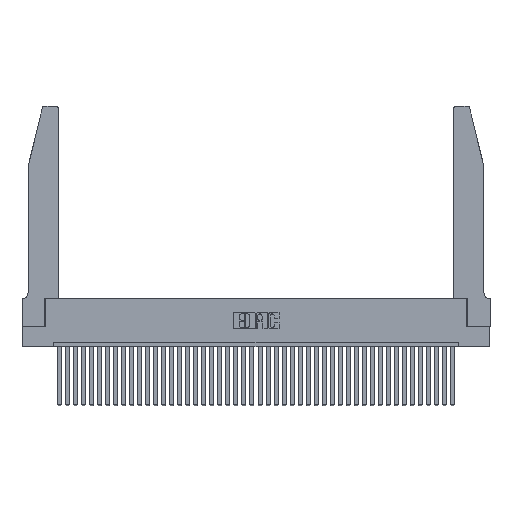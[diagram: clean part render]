
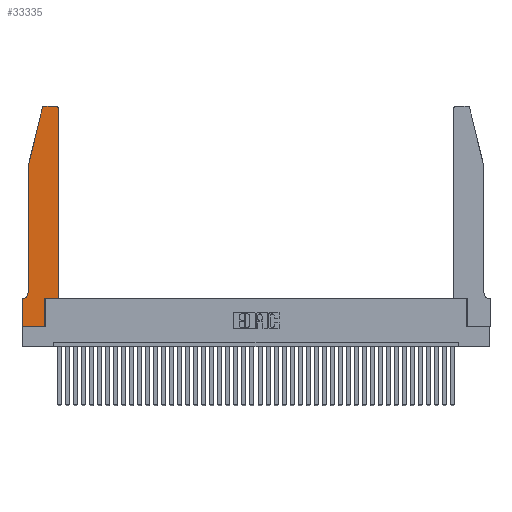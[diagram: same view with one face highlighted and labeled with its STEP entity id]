
A CAD part, top view. The second image highlights one B-rep face of the part: STEP entity #33335.
In plain terms, the highlighted planar face has unit normal (0, 0, 1).
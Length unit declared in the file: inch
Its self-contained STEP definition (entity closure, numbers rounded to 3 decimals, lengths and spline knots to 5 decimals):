
#812 = VERTEX_POINT ( 'NONE', #20611 ) ;
#815 = EDGE_CURVE ( 'NONE', #19528, #30898, #35516, .T. ) ;
#1488 = DIRECTION ( 'NONE',  ( -1., 0., 0. ) ) ;
#1812 = ORIENTED_EDGE ( 'NONE', *, *, #815, .T. ) ;
#2063 = CARTESIAN_POINT ( 'NONE',  ( 0.25487, 2.72718, 0.37 ) ) ;
#2068 = DIRECTION ( 'NONE',  ( 1., 0., 0. ) ) ;
#2325 = VECTOR ( 'NONE', #30915, 39.37008 ) ;
#2662 = CARTESIAN_POINT ( 'NONE',  ( 0.4505, 0.35, 0.37 ) ) ;
#3124 = CARTESIAN_POINT ( 'NONE',  ( 0.4505, 2.72, 0.37 ) ) ;
#3142 = AXIS2_PLACEMENT_3D ( 'NONE', #21998, #15865, #4964 ) ;
#3148 = EDGE_CURVE ( 'NONE', #8684, #4202, #26439, .T. ) ;
#3486 = CARTESIAN_POINT ( 'NONE',  ( 0.0755, 2., 0.37 ) ) ;
#3995 = EDGE_CURVE ( 'NONE', #35817, #8684, #11027, .T. ) ;
#4202 = VERTEX_POINT ( 'NONE', #2662 ) ;
#4600 = CARTESIAN_POINT ( 'NONE',  ( 0., 0.35, 0.37 ) ) ;
#4754 = VERTEX_POINT ( 'NONE', #38572 ) ;
#4964 = DIRECTION ( 'NONE',  ( -1., 0., 0. ) ) ;
#5086 = DIRECTION ( 'NONE',  ( 0., 0., 1. ) ) ;
#5355 = CARTESIAN_POINT ( 'NONE',  ( 0.0755, 0.35, 0.37 ) ) ;
#6106 = VECTOR ( 'NONE', #32020, 39.37008 ) ;
#6540 = CARTESIAN_POINT ( 'NONE',  ( 0.4505, 0.35, 0.37 ) ) ;
#6564 = DIRECTION ( 'NONE',  ( 1., 0., 0. ) ) ;
#7161 = CARTESIAN_POINT ( 'NONE',  ( 0.4505, 0.35, 0.37 ) ) ;
#7765 = EDGE_CURVE ( 'NONE', #4754, #24563, #22912, .T. ) ;
#8080 = VERTEX_POINT ( 'NONE', #11777 ) ;
#8684 = VERTEX_POINT ( 'NONE', #20878 ) ;
#9705 = LINE ( 'NONE', #7161, #41098 ) ;
#9980 = VECTOR ( 'NONE', #19160, 39.37008 ) ;
#10096 = ORIENTED_EDGE ( 'NONE', *, *, #23571, .T. ) ;
#11027 = LINE ( 'NONE', #32185, #9980 ) ;
#11777 = CARTESIAN_POINT ( 'NONE',  ( 0., 0., 0.37 ) ) ;
#12224 = CARTESIAN_POINT ( 'NONE',  ( 0., 0.35, 0.37 ) ) ;
#12759 = AXIS2_PLACEMENT_3D ( 'NONE', #28401, #19086, #18847 ) ;
#12921 = ORIENTED_EDGE ( 'NONE', *, *, #32391, .T. ) ;
#13575 = DIRECTION ( 'NONE',  ( 1., 0., 0. ) ) ;
#14182 = CARTESIAN_POINT ( 'NONE',  ( 0.0755, 2., 0.37 ) ) ;
#14288 = VECTOR ( 'NONE', #6564, 39.37008 ) ;
#15865 = DIRECTION ( 'NONE',  ( 0., 0., -1. ) ) ;
#15968 = EDGE_CURVE ( 'NONE', #29486, #812, #19612, .T. ) ;
#15982 = LINE ( 'NONE', #35861, #39393 ) ;
#16682 = ORIENTED_EDGE ( 'NONE', *, *, #32772, .T. ) ;
#17452 = VECTOR ( 'NONE', #38332, 39.37008 ) ;
#18021 = DIRECTION ( 'NONE',  ( 0., -1., 0. ) ) ;
#18697 = CARTESIAN_POINT ( 'NONE',  ( 0., 0., 0.37 ) ) ;
#18847 = DIRECTION ( 'NONE',  ( 1., 0., 0. ) ) ;
#19086 = DIRECTION ( 'NONE',  ( 0., 0., 1. ) ) ;
#19160 = DIRECTION ( 'NONE',  ( 0., 1., 0. ) ) ;
#19528 = VERTEX_POINT ( 'NONE', #32512 ) ;
#19612 = LINE ( 'NONE', #33725, #20686 ) ;
#19884 = VERTEX_POINT ( 'NONE', #3124 ) ;
#20611 = CARTESIAN_POINT ( 'NONE',  ( 0.0755, 0.42, 0.37 ) ) ;
#20686 = VECTOR ( 'NONE', #18021, 39.37008 ) ;
#20878 = CARTESIAN_POINT ( 'NONE',  ( 0.2865, 0.35, 0.37 ) ) ;
#21094 = ORIENTED_EDGE ( 'NONE', *, *, #29100, .T. ) ;
#21315 = ORIENTED_EDGE ( 'NONE', *, *, #27545, .T. ) ;
#21998 = CARTESIAN_POINT ( 'NONE',  ( 0.0055, 0.42, 0.37 ) ) ;
#22811 = FACE_OUTER_BOUND ( 'NONE', #30460, .T. ) ;
#22912 = LINE ( 'NONE', #5355, #6106 ) ;
#23571 = EDGE_CURVE ( 'NONE', #812, #4754, #39542, .T. ) ;
#24348 = CARTESIAN_POINT ( 'NONE',  ( 0., 0., 0.37 ) ) ;
#24454 = ORIENTED_EDGE ( 'NONE', *, *, #7765, .T. ) ;
#24563 = VERTEX_POINT ( 'NONE', #4600 ) ;
#24669 = CARTESIAN_POINT ( 'NONE',  ( 0.2865, 0., 0.37 ) ) ;
#26164 = AXIS2_PLACEMENT_3D ( 'NONE', #12224, #37521, #28185 ) ;
#26439 = LINE ( 'NONE', #6540, #39985 ) ;
#26876 = LINE ( 'NONE', #3486, #17452 ) ;
#27545 = EDGE_CURVE ( 'NONE', #8080, #35817, #32591, .T. ) ;
#27572 = LINE ( 'NONE', #24348, #2325 ) ;
#28185 = DIRECTION ( 'NONE',  ( 1., 0., 0. ) ) ;
#28315 = EDGE_CURVE ( 'NONE', #4202, #19884, #9705, .T. ) ;
#28401 = CARTESIAN_POINT ( 'NONE',  ( 0.4205, 2.72, 0.37 ) ) ;
#28623 = EDGE_CURVE ( 'NONE', #19884, #37465, #29539, .T. ) ;
#29100 = EDGE_CURVE ( 'NONE', #24563, #8080, #27572, .T. ) ;
#29207 = DIRECTION ( 'NONE',  ( 0., 1., 0. ) ) ;
#29486 = VERTEX_POINT ( 'NONE', #14182 ) ;
#29539 = CIRCLE ( 'NONE', #12759, 0.03 ) ;
#30460 = EDGE_LOOP ( 'NONE', ( #12921, #1812, #16682, #35519, #10096, #24454, #21094, #21315, #32044, #37725, #35417, #35436 ) ) ;
#30898 = VERTEX_POINT ( 'NONE', #2063 ) ;
#30907 = CARTESIAN_POINT ( 'NONE',  ( 0.284, 2.72, 0.37 ) ) ;
#30915 = DIRECTION ( 'NONE',  ( 0., -1., 0. ) ) ;
#32020 = DIRECTION ( 'NONE',  ( -1., 0., 0. ) ) ;
#32044 = ORIENTED_EDGE ( 'NONE', *, *, #3995, .T. ) ;
#32185 = CARTESIAN_POINT ( 'NONE',  ( 0.2865, 0.35, 0.37 ) ) ;
#32391 = EDGE_CURVE ( 'NONE', #37465, #19528, #15982, .T. ) ;
#32512 = CARTESIAN_POINT ( 'NONE',  ( 0.284, 2.75, 0.37 ) ) ;
#32591 = LINE ( 'NONE', #18697, #14288 ) ;
#32772 = EDGE_CURVE ( 'NONE', #30898, #29486, #26876, .T. ) ;
#33335 = ADVANCED_FACE ( 'NONE', ( #22811 ), #37917, .T. ) ;
#33725 = CARTESIAN_POINT ( 'NONE',  ( 0.0755, 2., 0.37 ) ) ;
#35417 = ORIENTED_EDGE ( 'NONE', *, *, #28315, .T. ) ;
#35436 = ORIENTED_EDGE ( 'NONE', *, *, #28623, .T. ) ;
#35516 = CIRCLE ( 'NONE', #37150, 0.03 ) ;
#35519 = ORIENTED_EDGE ( 'NONE', *, *, #15968, .T. ) ;
#35817 = VERTEX_POINT ( 'NONE', #24669 ) ;
#35861 = CARTESIAN_POINT ( 'NONE',  ( 0.2605, 2.75, 0.37 ) ) ;
#35947 = CARTESIAN_POINT ( 'NONE',  ( 0.4205, 2.75, 0.37 ) ) ;
#37150 = AXIS2_PLACEMENT_3D ( 'NONE', #30907, #5086, #2068 ) ;
#37465 = VERTEX_POINT ( 'NONE', #35947 ) ;
#37521 = DIRECTION ( 'NONE',  ( 0., 0., 1. ) ) ;
#37725 = ORIENTED_EDGE ( 'NONE', *, *, #3148, .T. ) ;
#37917 = PLANE ( 'NONE',  #26164 ) ;
#38332 = DIRECTION ( 'NONE',  ( -0.239, -0.971, 0. ) ) ;
#38572 = CARTESIAN_POINT ( 'NONE',  ( 0.0055, 0.35, 0.37 ) ) ;
#39393 = VECTOR ( 'NONE', #1488, 39.37008 ) ;
#39542 = CIRCLE ( 'NONE', #3142, 0.07 ) ;
#39985 = VECTOR ( 'NONE', #13575, 39.37008 ) ;
#41098 = VECTOR ( 'NONE', #29207, 39.37008 ) ;
